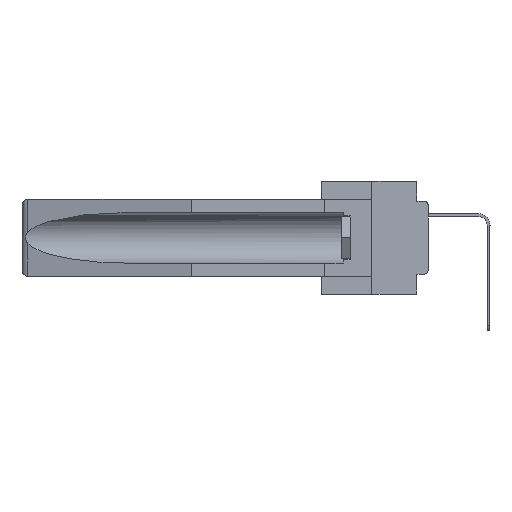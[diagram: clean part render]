
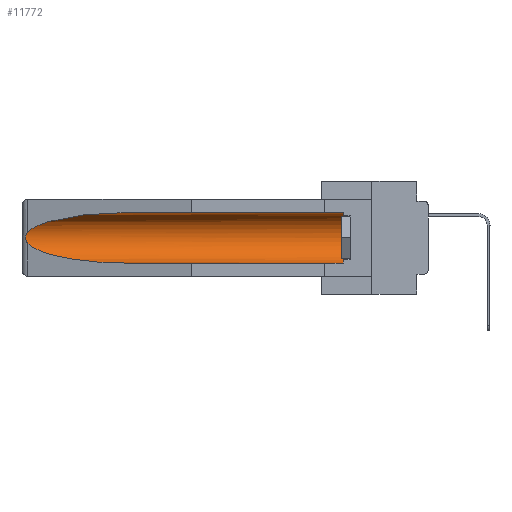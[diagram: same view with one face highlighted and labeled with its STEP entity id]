
A CAD part, left-side view. The second image highlights one B-rep face of the part: STEP entity #11772.
In plain terms, the highlighted cylindrical face has radius 2.857 mm (diameter 5.715 mm), a partial arc.
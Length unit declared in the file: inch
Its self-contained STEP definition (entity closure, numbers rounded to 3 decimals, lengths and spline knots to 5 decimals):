
#2346 = VERTEX_POINT ( 'NONE', #12734 ) ;
#2388 = CARTESIAN_POINT ( 'NONE',  ( 0.155, 0.126, -0.1715 ) ) ;
#3011 = CARTESIAN_POINT ( 'NONE',  ( 0.155, 1.07973, -0.059 ) ) ;
#3109 = CARTESIAN_POINT ( 'NONE',  ( 0.26537, 1.52718, -0.14972 ) ) ;
#3185 = EDGE_LOOP ( 'NONE', ( #8619, #15585, #20009, #25516, #4662, #13787 ) ) ;
#3839 = EDGE_CURVE ( 'NONE', #19999, #2346, #25835, .T. ) ;
#4140 = CARTESIAN_POINT ( 'NONE',  ( 0.155, 1.07973, -0.284 ) ) ;
#4662 = ORIENTED_EDGE ( 'NONE', *, *, #19374, .T. ) ;
#5701 = VERTEX_POINT ( 'NONE', #19229 ) ;
#6177 = CARTESIAN_POINT ( 'NONE',  ( 0.26537, 1.52718, -0.14972 ) ) ;
#7172 = CARTESIAN_POINT ( 'NONE',  ( 0.26537, 1.52718, -0.19328 ) ) ;
#7440 = CARTESIAN_POINT ( 'NONE',  ( 0.155, 1.07973, -0.059 ) ) ;
#8466 = CARTESIAN_POINT ( 'NONE',  ( 0.2673, 1.5327, -0.16383 ) ) ;
#8619 = ORIENTED_EDGE ( 'NONE', *, *, #3839, .T. ) ;
#8927 = CARTESIAN_POINT ( 'NONE',  ( 0.21114, 1.30732, -0.284 ) ) ;
#9017 = CARTESIAN_POINT ( 'NONE',  ( 0.25451, 1.48313, -0.24835 ) ) ;
#9254 = VECTOR ( 'NONE', #12586, 39.37008 ) ;
#9379 = EDGE_CURVE ( 'NONE', #2346, #28096, #17184, .T. ) ;
#9569 = CIRCLE ( 'NONE', #27481, 0.1125 ) ;
#10068 = FACE_OUTER_BOUND ( 'NONE', #3185, .T. ) ;
#10095 = VERTEX_POINT ( 'NONE', #26841 ) ;
#11539 = EDGE_CURVE ( 'NONE', #10095, #14754, #18510, .T. ) ;
#11772 = ADVANCED_FACE ( 'NONE', ( #10068 ), #27964, .F. ) ;
#12339 = CARTESIAN_POINT ( 'NONE',  ( 0.21114, 1.30732, -0.059 ) ) ;
#12586 = DIRECTION ( 'NONE',  ( 0., 1., 0. ) ) ;
#12734 = CARTESIAN_POINT ( 'NONE',  ( 0.26537, 1.52718, -0.14972 ) ) ;
#12766 = CARTESIAN_POINT ( 'NONE',  ( 0.155, -0.30754, -0.1715 ) ) ;
#13268 = CARTESIAN_POINT ( 'NONE',  ( 0.2673, 1.53269, -0.17917 ) ) ;
#13426 = EDGE_CURVE ( 'NONE', #5701, #19999, #27862, .T. ) ;
#13787 = ORIENTED_EDGE ( 'NONE', *, *, #13426, .T. ) ;
#14474 = CARTESIAN_POINT ( 'NONE',  ( 0.25451, 1.48313, -0.09465 ) ) ;
#14754 = VERTEX_POINT ( 'NONE', #4140 ) ;
#14970 = DIRECTION ( 'NONE',  ( 0., 1., 0. ) ) ;
#15289 = CARTESIAN_POINT ( 'NONE',  ( 0.26597, 1.5296, -0.19026 ) ) ;
#15585 = ORIENTED_EDGE ( 'NONE', *, *, #9379, .T. ) ;
#15916 = DIRECTION ( 'NONE',  ( 0., -1., 0. ) ) ;
#17070 = CARTESIAN_POINT ( 'NONE',  ( 0.155, -0.30754, -0.059 ) ) ;
#17184 = B_SPLINE_CURVE_WITH_KNOTS ( 'NONE', 3,
 ( #6177, #21890, #19919, #8466, #17666, #22078, #13268, #24430, #15289, #24145 ),
 .UNSPECIFIED., .F., .F.,
 ( 4, 2, 2, 2, 4 ),
 ( 0., 0.00029, 0.00058, 0.00087, 0.00117 ),
 .UNSPECIFIED. ) ;
#17666 = CARTESIAN_POINT ( 'NONE',  ( 0.2675, 1.53308, -0.16763 ) ) ;
#18072 = DIRECTION ( 'NONE',  ( 0., 0., 1. ) ) ;
#18510 = LINE ( 'NONE', #18826, #19559 ) ;
#18826 = CARTESIAN_POINT ( 'NONE',  ( 0.155, -0.30754, -0.284 ) ) ;
#19229 = CARTESIAN_POINT ( 'NONE',  ( 0.155, 0.126, -0.059 ) ) ;
#19374 = EDGE_CURVE ( 'NONE', #10095, #5701, #9569, .T. ) ;
#19527 = CARTESIAN_POINT ( 'NONE',  ( 0.155, 1.07973, -0.284 ) ) ;
#19559 = VECTOR ( 'NONE', #27748, 39.37008 ) ;
#19722 = EDGE_CURVE ( 'NONE', #28096, #14754, #20610, .T. ) ;
#19919 = CARTESIAN_POINT ( 'NONE',  ( 0.26654, 1.53092, -0.15636 ) ) ;
#19999 = VERTEX_POINT ( 'NONE', #7440 ) ;
#20009 = ORIENTED_EDGE ( 'NONE', *, *, #19722, .T. ) ;
#20610 =( BOUNDED_CURVE ( )  B_SPLINE_CURVE ( 3, ( #22374, #9017, #8927, #19527 ),
 .UNSPECIFIED., .F., .F. ) 
 B_SPLINE_CURVE_WITH_KNOTS ( ( 4, 4 ),
 ( 0.1948, 1.5708 ),
 .UNSPECIFIED. ) 
 CURVE ( )  GEOMETRIC_REPRESENTATION_ITEM ( )  RATIONAL_B_SPLINE_CURVE ( ( 1., 0.848, 0.848, 1. ) ) 
 REPRESENTATION_ITEM ( '' )  );
#21890 = CARTESIAN_POINT ( 'NONE',  ( 0.26597, 1.52961, -0.15275 ) ) ;
#22078 = CARTESIAN_POINT ( 'NONE',  ( 0.2675, 1.53308, -0.17534 ) ) ;
#22374 = CARTESIAN_POINT ( 'NONE',  ( 0.26537, 1.52718, -0.19328 ) ) ;
#22755 = AXIS2_PLACEMENT_3D ( 'NONE', #12766, #14970, #23551 ) ;
#23551 = DIRECTION ( 'NONE',  ( 0., 0., 1. ) ) ;
#24145 = CARTESIAN_POINT ( 'NONE',  ( 0.26537, 1.52718, -0.19328 ) ) ;
#24430 = CARTESIAN_POINT ( 'NONE',  ( 0.26655, 1.53094, -0.18657 ) ) ;
#25516 = ORIENTED_EDGE ( 'NONE', *, *, #11539, .F. ) ;
#25835 =( BOUNDED_CURVE ( )  B_SPLINE_CURVE ( 3, ( #3011, #12339, #14474, #3109 ),
 .UNSPECIFIED., .F., .F. ) 
 B_SPLINE_CURVE_WITH_KNOTS ( ( 4, 4 ),
 ( 4.71239, 6.08839 ),
 .UNSPECIFIED. ) 
 CURVE ( )  GEOMETRIC_REPRESENTATION_ITEM ( )  RATIONAL_B_SPLINE_CURVE ( ( 1., 0.848, 0.848, 1. ) ) 
 REPRESENTATION_ITEM ( '' )  );
#26841 = CARTESIAN_POINT ( 'NONE',  ( 0.155, 0.126, -0.284 ) ) ;
#27481 = AXIS2_PLACEMENT_3D ( 'NONE', #2388, #15916, #18072 ) ;
#27748 = DIRECTION ( 'NONE',  ( 0., 1., 0. ) ) ;
#27862 = LINE ( 'NONE', #17070, #9254 ) ;
#27964 = CYLINDRICAL_SURFACE ( 'NONE', #22755, 0.1125 ) ;
#28096 = VERTEX_POINT ( 'NONE', #7172 ) ;
